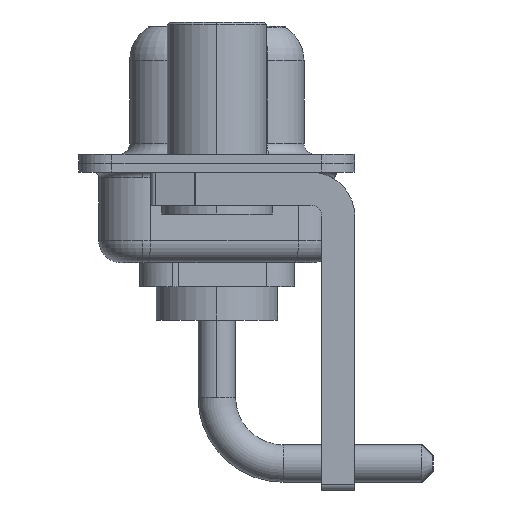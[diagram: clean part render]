
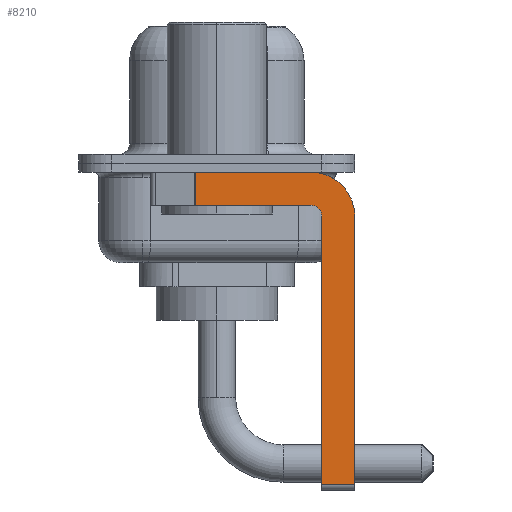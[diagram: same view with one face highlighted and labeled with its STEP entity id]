
A CAD part, left-side view. The second image highlights one B-rep face of the part: STEP entity #8210.
In plain terms, the highlighted planar face has unit normal (-1, 0, 0).
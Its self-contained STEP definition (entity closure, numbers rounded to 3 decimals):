
#195 = ORIENTED_EDGE ( 'NONE', *, *, #3472, .T. ) ;
#554 = DIRECTION ( 'NONE',  ( 0., 0., -1. ) ) ;
#630 = LINE ( 'NONE', #1783, #10768 ) ;
#825 = CARTESIAN_POINT ( 'NONE',  ( -2.9, -6.25, -2.4 ) ) ;
#1071 = CARTESIAN_POINT ( 'NONE',  ( -2.9, 0.978, -1.9 ) ) ;
#1120 = VECTOR ( 'NONE', #11025, 1000. ) ;
#1181 = CARTESIAN_POINT ( 'NONE',  ( -2.9, -4.75, -14.8 ) ) ;
#1396 = ORIENTED_EDGE ( 'NONE', *, *, #16237, .F. ) ;
#1757 = VERTEX_POINT ( 'NONE', #825 ) ;
#1783 = CARTESIAN_POINT ( 'NONE',  ( -2.9, -6.25, -2.4 ) ) ;
#1974 = VERTEX_POINT ( 'NONE', #6362 ) ;
#2002 = EDGE_CURVE ( 'NONE', #10791, #3638, #12363, .T. ) ;
#2177 = ORIENTED_EDGE ( 'NONE', *, *, #10075, .F. ) ;
#2340 = ORIENTED_EDGE ( 'NONE', *, *, #13321, .F. ) ;
#2553 = AXIS2_PLACEMENT_3D ( 'NONE', #8542, #12329, #4430 ) ;
#2601 = DIRECTION ( 'NONE',  ( 0., -1., 0. ) ) ;
#3097 = AXIS2_PLACEMENT_3D ( 'NONE', #13314, #4663, #12247 ) ;
#3246 = CARTESIAN_POINT ( 'NONE',  ( -2.9, -4.75, -2.4 ) ) ;
#3275 = EDGE_CURVE ( 'NONE', #15110, #11435, #5812, .T. ) ;
#3472 = EDGE_CURVE ( 'NONE', #5577, #1974, #9860, .T. ) ;
#3638 = VERTEX_POINT ( 'NONE', #11676 ) ;
#3650 = FACE_OUTER_BOUND ( 'NONE', #7080, .T. ) ;
#3733 = CARTESIAN_POINT ( 'NONE',  ( -2.9, 0.978, -0.4 ) ) ;
#4430 = DIRECTION ( 'NONE',  ( 0., 0., 1. ) ) ;
#4538 = ORIENTED_EDGE ( 'NONE', *, *, #8998, .F. ) ;
#4663 = DIRECTION ( 'NONE',  ( 1., 0., 0. ) ) ;
#4970 = LINE ( 'NONE', #7280, #12383 ) ;
#5577 = VERTEX_POINT ( 'NONE', #12551 ) ;
#5812 = CIRCLE ( 'NONE', #2553, 0.5 ) ;
#5996 = CIRCLE ( 'NONE', #3097, 2. ) ;
#5999 = CARTESIAN_POINT ( 'NONE',  ( -2.9, -4.25, -1.9 ) ) ;
#6082 = CARTESIAN_POINT ( 'NONE',  ( -2.9, -4.25, -1.9 ) ) ;
#6362 = CARTESIAN_POINT ( 'NONE',  ( -2.9, -6.25, -14.55 ) ) ;
#7080 = EDGE_LOOP ( 'NONE', ( #2340, #13587, #1396, #11612, #4538, #195, #9254, #2177 ) ) ;
#7280 = CARTESIAN_POINT ( 'NONE',  ( -2.9, 3., -0.4 ) ) ;
#7292 = DIRECTION ( 'NONE',  ( 1., 0., 0. ) ) ;
#7381 = VECTOR ( 'NONE', #12514, 1000. ) ;
#7537 = PLANE ( 'NONE',  #13581 ) ;
#8210 = ADVANCED_FACE ( 'NONE', ( #3650 ), #7537, .F. ) ;
#8366 = VECTOR ( 'NONE', #2601, 1000. ) ;
#8470 = LINE ( 'NONE', #5999, #1120 ) ;
#8542 = CARTESIAN_POINT ( 'NONE',  ( -2.9, -4.25, -2.4 ) ) ;
#8702 = CARTESIAN_POINT ( 'NONE',  ( -2.9, -4.25, -0.4 ) ) ;
#8781 = DIRECTION ( 'NONE',  ( 0., 0., 1. ) ) ;
#8916 = VERTEX_POINT ( 'NONE', #8702 ) ;
#8998 = EDGE_CURVE ( 'NONE', #5577, #15110, #15049, .T. ) ;
#9254 = ORIENTED_EDGE ( 'NONE', *, *, #11305, .F. ) ;
#9860 = LINE ( 'NONE', #12478, #8366 ) ;
#10001 = DIRECTION ( 'NONE',  ( 0., -1., 0. ) ) ;
#10075 = EDGE_CURVE ( 'NONE', #8916, #1757, #5996, .T. ) ;
#10768 = VECTOR ( 'NONE', #554, 1000. ) ;
#10791 = VERTEX_POINT ( 'NONE', #3733 ) ;
#11025 = DIRECTION ( 'NONE',  ( 0., 1., 0. ) ) ;
#11095 = CARTESIAN_POINT ( 'NONE',  ( -2.9, -4.25, -2.4 ) ) ;
#11305 = EDGE_CURVE ( 'NONE', #1757, #1974, #630, .T. ) ;
#11435 = VERTEX_POINT ( 'NONE', #6082 ) ;
#11612 = ORIENTED_EDGE ( 'NONE', *, *, #3275, .F. ) ;
#11676 = CARTESIAN_POINT ( 'NONE',  ( -2.9, 0.978, -1.9 ) ) ;
#12247 = DIRECTION ( 'NONE',  ( 0., 0., -1. ) ) ;
#12279 = VECTOR ( 'NONE', #8781, 1000. ) ;
#12329 = DIRECTION ( 'NONE',  ( -1., 0., 0. ) ) ;
#12363 = LINE ( 'NONE', #1071, #7381 ) ;
#12383 = VECTOR ( 'NONE', #10001, 1000. ) ;
#12465 = DIRECTION ( 'NONE',  ( 0., 0., -1. ) ) ;
#12478 = CARTESIAN_POINT ( 'NONE',  ( -2.9, -4.25, -14.55 ) ) ;
#12514 = DIRECTION ( 'NONE',  ( 0., 0., -1. ) ) ;
#12551 = CARTESIAN_POINT ( 'NONE',  ( -2.9, -4.75, -14.55 ) ) ;
#13314 = CARTESIAN_POINT ( 'NONE',  ( -2.9, -4.25, -2.4 ) ) ;
#13321 = EDGE_CURVE ( 'NONE', #10791, #8916, #4970, .T. ) ;
#13581 = AXIS2_PLACEMENT_3D ( 'NONE', #11095, #7292, #12465 ) ;
#13587 = ORIENTED_EDGE ( 'NONE', *, *, #2002, .T. ) ;
#15049 = LINE ( 'NONE', #1181, #12279 ) ;
#15110 = VERTEX_POINT ( 'NONE', #3246 ) ;
#16237 = EDGE_CURVE ( 'NONE', #11435, #3638, #8470, .T. ) ;
